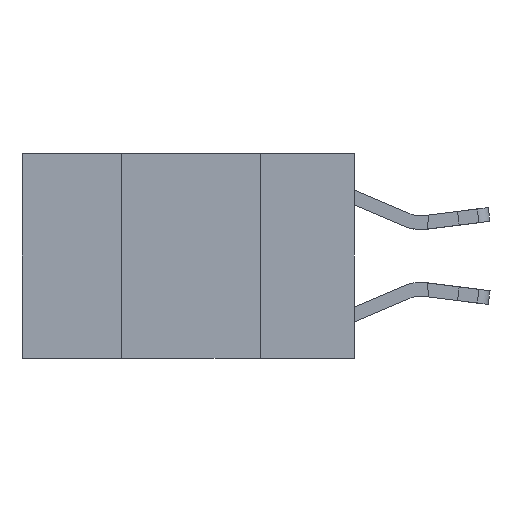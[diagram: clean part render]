
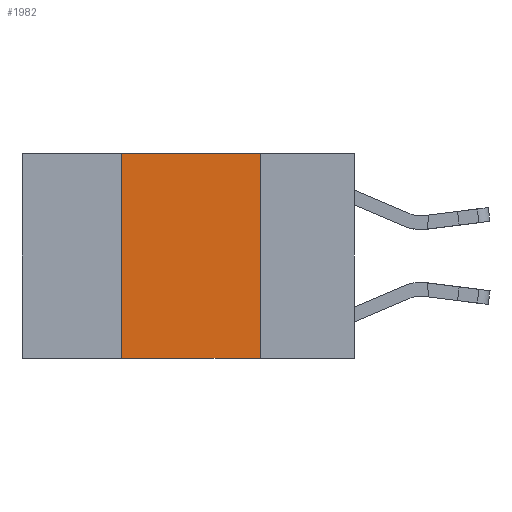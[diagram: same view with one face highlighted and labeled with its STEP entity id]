
A CAD part, left-side view. The second image highlights one B-rep face of the part: STEP entity #1982.
In plain terms, the highlighted planar face has unit normal (-1, 0, 0).
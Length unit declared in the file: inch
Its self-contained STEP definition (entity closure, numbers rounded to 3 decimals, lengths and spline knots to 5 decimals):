
#437 = CARTESIAN_POINT ( 'NONE',  ( 0., 0.42, 0. ) ) ;
#789 = CARTESIAN_POINT ( 'NONE',  ( 0., 0.42, 0. ) ) ;
#1048 = VECTOR ( 'NONE', #3637, 39.37008 ) ;
#1879 = ORIENTED_EDGE ( 'NONE', *, *, #3981, .T. ) ;
#1982 = ADVANCED_FACE ( 'NONE', ( #15290 ), #2314, .F. ) ;
#2215 = DIRECTION ( 'NONE',  ( 0., -1., 0. ) ) ;
#2314 = PLANE ( 'NONE',  #8821 ) ;
#2624 = EDGE_LOOP ( 'NONE', ( #9369, #5700, #9857, #1879 ) ) ;
#2917 = VERTEX_POINT ( 'NONE', #3079 ) ;
#3079 = CARTESIAN_POINT ( 'NONE',  ( 0., 0.42, -0.37 ) ) ;
#3637 = DIRECTION ( 'NONE',  ( 0., 0., -1. ) ) ;
#3969 = DIRECTION ( 'NONE',  ( 1., 0., 0. ) ) ;
#3970 = LINE ( 'NONE', #4745, #15826 ) ;
#3981 = EDGE_CURVE ( 'NONE', #2917, #11555, #16583, .T. ) ;
#4745 = CARTESIAN_POINT ( 'NONE',  ( 0., 0.6, 0. ) ) ;
#5234 = CARTESIAN_POINT ( 'NONE',  ( 0., 0.17, 0. ) ) ;
#5456 = LINE ( 'NONE', #5234, #1048 ) ;
#5586 = EDGE_CURVE ( 'NONE', #2917, #11137, #18554, .T. ) ;
#5692 = DIRECTION ( 'NONE',  ( 0., 0., 1. ) ) ;
#5700 = ORIENTED_EDGE ( 'NONE', *, *, #14091, .F. ) ;
#6362 = DIRECTION ( 'NONE',  ( 0., -1., 0. ) ) ;
#7060 = CARTESIAN_POINT ( 'NONE',  ( 0., 0.6, -0.37 ) ) ;
#8821 = AXIS2_PLACEMENT_3D ( 'NONE', #13242, #3969, #14861 ) ;
#9369 = ORIENTED_EDGE ( 'NONE', *, *, #10195, .F. ) ;
#9857 = ORIENTED_EDGE ( 'NONE', *, *, #5586, .F. ) ;
#10195 = EDGE_CURVE ( 'NONE', #18701, #11555, #5456, .T. ) ;
#11137 = VERTEX_POINT ( 'NONE', #437 ) ;
#11555 = VERTEX_POINT ( 'NONE', #16907 ) ;
#13242 = CARTESIAN_POINT ( 'NONE',  ( 0., 0.6, 0. ) ) ;
#14091 = EDGE_CURVE ( 'NONE', #11137, #18701, #3970, .T. ) ;
#14688 = VECTOR ( 'NONE', #5692, 39.37008 ) ;
#14861 = DIRECTION ( 'NONE',  ( 0., 0., -1. ) ) ;
#15290 = FACE_OUTER_BOUND ( 'NONE', #2624, .T. ) ;
#15826 = VECTOR ( 'NONE', #6362, 39.37008 ) ;
#16124 = VECTOR ( 'NONE', #2215, 39.37008 ) ;
#16583 = LINE ( 'NONE', #7060, #16124 ) ;
#16863 = CARTESIAN_POINT ( 'NONE',  ( 0., 0.17, 0. ) ) ;
#16907 = CARTESIAN_POINT ( 'NONE',  ( 0., 0.17, -0.37 ) ) ;
#18554 = LINE ( 'NONE', #789, #14688 ) ;
#18701 = VERTEX_POINT ( 'NONE', #16863 ) ;
